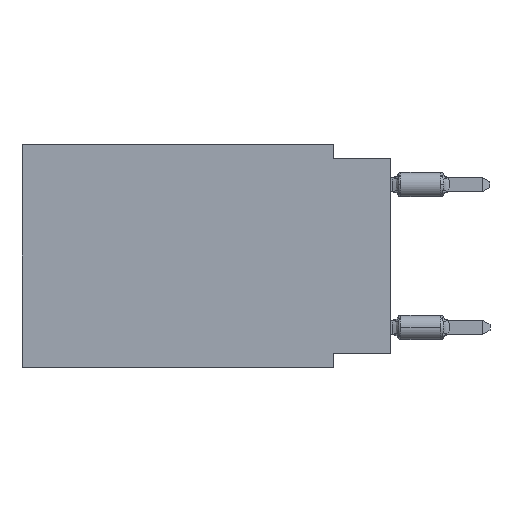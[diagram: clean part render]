
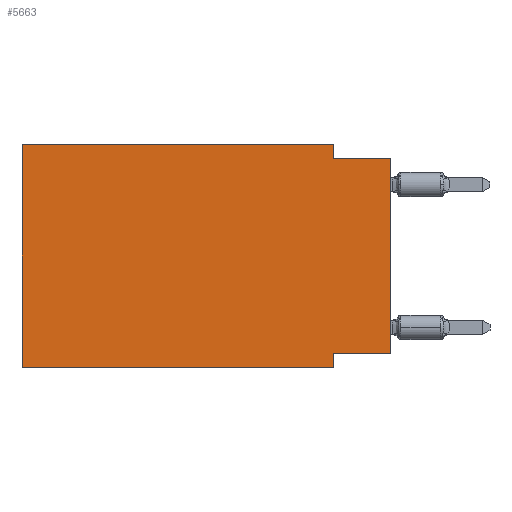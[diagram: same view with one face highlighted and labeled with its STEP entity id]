
A CAD part, left-side view. The second image highlights one B-rep face of the part: STEP entity #5663.
In plain terms, the highlighted planar face has unit normal (-1, 0, 0).
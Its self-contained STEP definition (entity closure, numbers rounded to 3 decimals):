
#124 = VERTEX_POINT ( 'NONE', #861 ) ;
#737 = CARTESIAN_POINT ( 'NONE',  ( 0., 16.383, 0. ) ) ;
#861 = CARTESIAN_POINT ( 'NONE',  ( 0., 2.54, 0. ) ) ;
#1343 = DIRECTION ( 'NONE',  ( 0., 1., 0. ) ) ;
#1394 = CARTESIAN_POINT ( 'NONE',  ( 0., 16.383, 0. ) ) ;
#1690 = CARTESIAN_POINT ( 'NONE',  ( 0., 0., -9.271 ) ) ;
#1694 = VECTOR ( 'NONE', #9241, 1000. ) ;
#1774 = AXIS2_PLACEMENT_3D ( 'NONE', #15663, #7492, #6193 ) ;
#2836 = LINE ( 'NONE', #16120, #1694 ) ;
#3324 = CARTESIAN_POINT ( 'NONE',  ( 0., 2.54, -9.906 ) ) ;
#3428 = DIRECTION ( 'NONE',  ( 0., -1., 0. ) ) ;
#3638 = ORIENTED_EDGE ( 'NONE', *, *, #6960, .F. ) ;
#3642 = VECTOR ( 'NONE', #3714, 1000. ) ;
#3714 = DIRECTION ( 'NONE',  ( 0., -1., 0. ) ) ;
#3805 = ORIENTED_EDGE ( 'NONE', *, *, #12577, .T. ) ;
#3806 = LINE ( 'NONE', #11782, #3642 ) ;
#3842 = VECTOR ( 'NONE', #3428, 1000. ) ;
#3994 = CARTESIAN_POINT ( 'NONE',  ( 0., 2.54, 0. ) ) ;
#4352 = CARTESIAN_POINT ( 'NONE',  ( 0., 0., -0.635 ) ) ;
#4393 = ORIENTED_EDGE ( 'NONE', *, *, #9388, .F. ) ;
#4807 = LINE ( 'NONE', #737, #3842 ) ;
#4858 = EDGE_LOOP ( 'NONE', ( #12447, #15828, #7330, #12236, #12947, #3805, #4393, #3638 ) ) ;
#4903 = VECTOR ( 'NONE', #1343, 1000. ) ;
#5011 = DIRECTION ( 'NONE',  ( 0., 0., -1. ) ) ;
#5215 = LINE ( 'NONE', #1394, #15559 ) ;
#5663 = ADVANCED_FACE ( 'NONE', ( #17131 ), #10103, .F. ) ;
#5877 = VERTEX_POINT ( 'NONE', #14011 ) ;
#6064 = CARTESIAN_POINT ( 'NONE',  ( 0., 0., -0.635 ) ) ;
#6091 = DIRECTION ( 'NONE',  ( 0., 0., -1. ) ) ;
#6193 = DIRECTION ( 'NONE',  ( 0., 0., -1. ) ) ;
#6487 = EDGE_CURVE ( 'NONE', #14007, #11866, #15463, .T. ) ;
#6751 = VERTEX_POINT ( 'NONE', #16621 ) ;
#6960 = EDGE_CURVE ( 'NONE', #6751, #12289, #9407, .T. ) ;
#7330 = ORIENTED_EDGE ( 'NONE', *, *, #10014, .F. ) ;
#7492 = DIRECTION ( 'NONE',  ( 1., 0., 0. ) ) ;
#8651 = VECTOR ( 'NONE', #6091, 1000. ) ;
#9241 = DIRECTION ( 'NONE',  ( 0., 0., 1. ) ) ;
#9351 = VERTEX_POINT ( 'NONE', #10480 ) ;
#9388 = EDGE_CURVE ( 'NONE', #12289, #13597, #10300, .T. ) ;
#9407 = LINE ( 'NONE', #1690, #4903 ) ;
#10014 = EDGE_CURVE ( 'NONE', #124, #14007, #16769, .T. ) ;
#10103 = PLANE ( 'NONE',  #1774 ) ;
#10300 = LINE ( 'NONE', #11778, #14034 ) ;
#10414 = DIRECTION ( 'NONE',  ( 0., 0., 1. ) ) ;
#10480 = CARTESIAN_POINT ( 'NONE',  ( 0., 16.383, -9.906 ) ) ;
#11512 = CARTESIAN_POINT ( 'NONE',  ( 0., 2.54, -0.635 ) ) ;
#11778 = CARTESIAN_POINT ( 'NONE',  ( 0., 2.54, -9.906 ) ) ;
#11782 = CARTESIAN_POINT ( 'NONE',  ( 0., 16.383, -9.906 ) ) ;
#11866 = VERTEX_POINT ( 'NONE', #4352 ) ;
#11958 = EDGE_CURVE ( 'NONE', #6751, #11866, #2836, .T. ) ;
#12180 = EDGE_CURVE ( 'NONE', #9351, #5877, #5215, .T. ) ;
#12236 = ORIENTED_EDGE ( 'NONE', *, *, #14380, .F. ) ;
#12289 = VERTEX_POINT ( 'NONE', #14868 ) ;
#12447 = ORIENTED_EDGE ( 'NONE', *, *, #11958, .T. ) ;
#12577 = EDGE_CURVE ( 'NONE', #9351, #13597, #3806, .T. ) ;
#12947 = ORIENTED_EDGE ( 'NONE', *, *, #12180, .F. ) ;
#13597 = VERTEX_POINT ( 'NONE', #3324 ) ;
#14007 = VERTEX_POINT ( 'NONE', #11512 ) ;
#14011 = CARTESIAN_POINT ( 'NONE',  ( 0., 16.383, 0. ) ) ;
#14034 = VECTOR ( 'NONE', #5011, 1000. ) ;
#14380 = EDGE_CURVE ( 'NONE', #5877, #124, #4807, .T. ) ;
#14868 = CARTESIAN_POINT ( 'NONE',  ( 0., 2.54, -9.271 ) ) ;
#15463 = LINE ( 'NONE', #6064, #16521 ) ;
#15559 = VECTOR ( 'NONE', #10414, 1000. ) ;
#15663 = CARTESIAN_POINT ( 'NONE',  ( 0., 16.383, 0. ) ) ;
#15828 = ORIENTED_EDGE ( 'NONE', *, *, #6487, .F. ) ;
#16120 = CARTESIAN_POINT ( 'NONE',  ( 0., 0., 0. ) ) ;
#16521 = VECTOR ( 'NONE', #16917, 1000. ) ;
#16621 = CARTESIAN_POINT ( 'NONE',  ( 0., 0., -9.271 ) ) ;
#16769 = LINE ( 'NONE', #3994, #8651 ) ;
#16917 = DIRECTION ( 'NONE',  ( 0., -1., 0. ) ) ;
#17131 = FACE_OUTER_BOUND ( 'NONE', #4858, .T. ) ;
